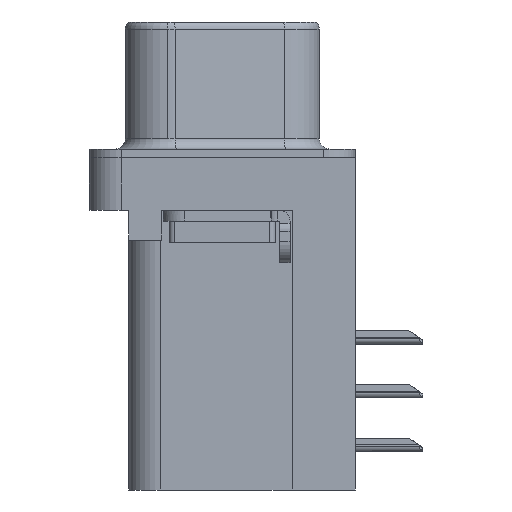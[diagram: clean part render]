
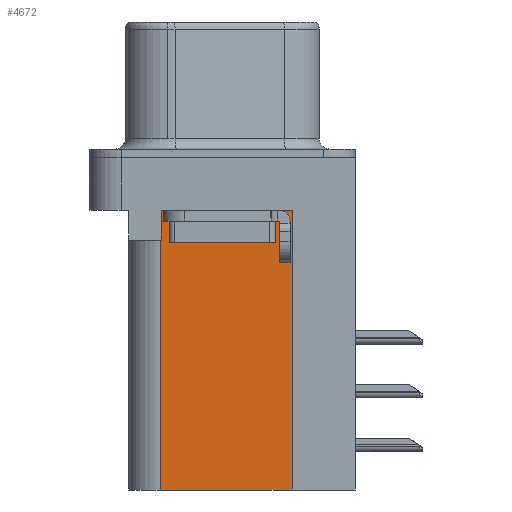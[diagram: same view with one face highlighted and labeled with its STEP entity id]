
A CAD part, left-side view. The second image highlights one B-rep face of the part: STEP entity #4672.
In plain terms, the highlighted planar face has unit normal (-1, 0, 0).
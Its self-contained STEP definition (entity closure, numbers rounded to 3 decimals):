
#1108 = VECTOR ( 'NONE', #2478, 1000. ) ;
#2478 = DIRECTION ( 'NONE',  ( 0., 0., 1. ) ) ;
#3046 = VERTEX_POINT ( 'NONE', #7744 ) ;
#3984 = DIRECTION ( 'NONE',  ( 0., 1., 0. ) ) ;
#4672 = ADVANCED_FACE ( 'NONE', ( #6986 ), #30820, .F. ) ;
#5238 = ORIENTED_EDGE ( 'NONE', *, *, #23530, .T. ) ;
#5940 = VECTOR ( 'NONE', #12898, 1000. ) ;
#6986 = FACE_OUTER_BOUND ( 'NONE', #18735, .T. ) ;
#7744 = CARTESIAN_POINT ( 'NONE',  ( 3.79, -3.295, -2.5 ) ) ;
#8271 = CARTESIAN_POINT ( 'NONE',  ( 3.79, -3.295, -15.7 ) ) ;
#9135 = CARTESIAN_POINT ( 'NONE',  ( 3.79, -3.295, -15.7 ) ) ;
#9446 = CARTESIAN_POINT ( 'NONE',  ( 3.79, 2.925, -15.7 ) ) ;
#10237 = VERTEX_POINT ( 'NONE', #27100 ) ;
#10298 = LINE ( 'NONE', #8271, #31108 ) ;
#10919 = CARTESIAN_POINT ( 'NONE',  ( 3.79, -3.295, -15.7 ) ) ;
#12206 = EDGE_CURVE ( 'NONE', #31833, #10237, #29106, .T. ) ;
#12898 = DIRECTION ( 'NONE',  ( 0., 1., 0. ) ) ;
#13204 = LINE ( 'NONE', #10919, #19472 ) ;
#13840 = LINE ( 'NONE', #26430, #5940 ) ;
#16839 = AXIS2_PLACEMENT_3D ( 'NONE', #9135, #22529, #33562 ) ;
#18051 = ORIENTED_EDGE ( 'NONE', *, *, #33595, .F. ) ;
#18136 = CARTESIAN_POINT ( 'NONE',  ( 3.79, 2.925, -3.9 ) ) ;
#18212 = CARTESIAN_POINT ( 'NONE',  ( 3.79, 2.895, -3.9 ) ) ;
#18735 = EDGE_LOOP ( 'NONE', ( #19511, #27644, #27258, #18051, #24774, #5238 ) ) ;
#19472 = VECTOR ( 'NONE', #27140, 1000. ) ;
#19511 = ORIENTED_EDGE ( 'NONE', *, *, #31788, .T. ) ;
#20330 = VERTEX_POINT ( 'NONE', #18136 ) ;
#22529 = DIRECTION ( 'NONE',  ( 1., 0., 0. ) ) ;
#22636 = CARTESIAN_POINT ( 'NONE',  ( 3.79, -3.295, -15.7 ) ) ;
#22672 = LINE ( 'NONE', #34985, #1108 ) ;
#22854 = CARTESIAN_POINT ( 'NONE',  ( 3.79, -3.295, -2.5 ) ) ;
#23114 = VERTEX_POINT ( 'NONE', #9446 ) ;
#23530 = EDGE_CURVE ( 'NONE', #24431, #3046, #10298, .T. ) ;
#24431 = VERTEX_POINT ( 'NONE', #22636 ) ;
#24774 = ORIENTED_EDGE ( 'NONE', *, *, #29910, .F. ) ;
#25722 = CARTESIAN_POINT ( 'NONE',  ( 3.79, 2.895, -2.5 ) ) ;
#25897 = EDGE_CURVE ( 'NONE', #10237, #20330, #13840, .T. ) ;
#26430 = CARTESIAN_POINT ( 'NONE',  ( 3.79, 0., -3.9 ) ) ;
#26724 = LINE ( 'NONE', #22854, #27578 ) ;
#27100 = CARTESIAN_POINT ( 'NONE',  ( 3.79, 2.895, -3.9 ) ) ;
#27140 = DIRECTION ( 'NONE',  ( 0., 1., 0. ) ) ;
#27258 = ORIENTED_EDGE ( 'NONE', *, *, #25897, .T. ) ;
#27578 = VECTOR ( 'NONE', #3984, 1000. ) ;
#27644 = ORIENTED_EDGE ( 'NONE', *, *, #12206, .T. ) ;
#29106 = LINE ( 'NONE', #18212, #29955 ) ;
#29910 = EDGE_CURVE ( 'NONE', #24431, #23114, #13204, .T. ) ;
#29955 = VECTOR ( 'NONE', #34606, 1000. ) ;
#30027 = DIRECTION ( 'NONE',  ( 0., 0., 1. ) ) ;
#30820 = PLANE ( 'NONE',  #16839 ) ;
#31108 = VECTOR ( 'NONE', #30027, 1000. ) ;
#31788 = EDGE_CURVE ( 'NONE', #3046, #31833, #26724, .T. ) ;
#31833 = VERTEX_POINT ( 'NONE', #25722 ) ;
#33562 = DIRECTION ( 'NONE',  ( 0., 0., -1. ) ) ;
#33595 = EDGE_CURVE ( 'NONE', #23114, #20330, #22672, .T. ) ;
#34606 = DIRECTION ( 'NONE',  ( 0., 0., -1. ) ) ;
#34985 = CARTESIAN_POINT ( 'NONE',  ( 3.79, 2.925, -15.7 ) ) ;
